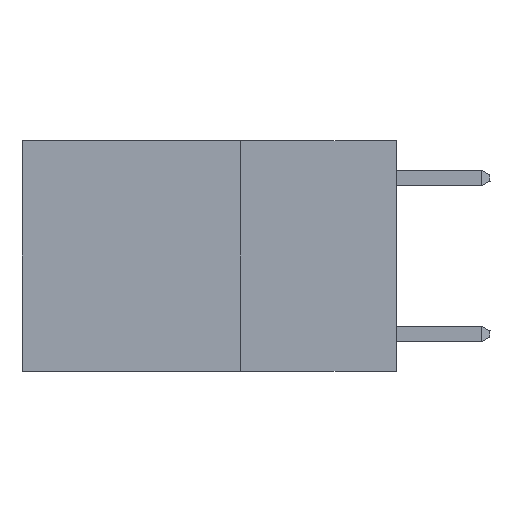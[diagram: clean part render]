
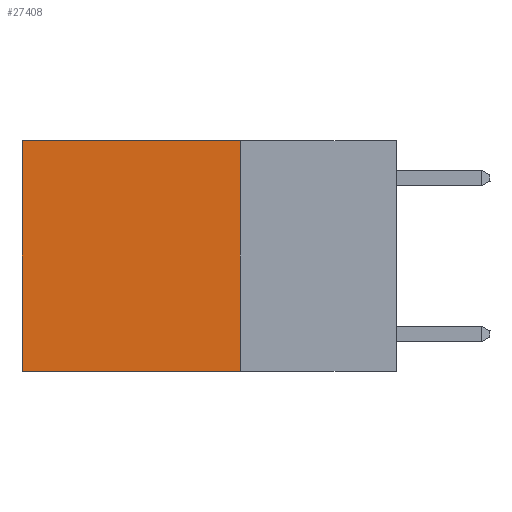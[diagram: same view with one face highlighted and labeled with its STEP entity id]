
A CAD part, left-side view. The second image highlights one B-rep face of the part: STEP entity #27408.
In plain terms, the highlighted planar face has unit normal (-1, 0, 0).
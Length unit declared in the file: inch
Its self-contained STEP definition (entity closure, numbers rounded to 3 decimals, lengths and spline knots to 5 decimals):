
#309 = VECTOR ( 'NONE', #12579, 39.37008 ) ;
#329 = DIRECTION ( 'NONE',  ( 1., 0., 0. ) ) ;
#1206 = VECTOR ( 'NONE', #25152, 39.37008 ) ;
#2781 = EDGE_CURVE ( 'NONE', #13304, #29203, #20302, .T. ) ;
#4089 = EDGE_CURVE ( 'NONE', #20739, #18573, #15946, .T. ) ;
#4998 = PLANE ( 'NONE',  #27198 ) ;
#7076 = CARTESIAN_POINT ( 'NONE',  ( 0.2625, 0.25, 0. ) ) ;
#8182 = ORIENTED_EDGE ( 'NONE', *, *, #2781, .T. ) ;
#8231 = LINE ( 'NONE', #8534, #309 ) ;
#8534 = CARTESIAN_POINT ( 'NONE',  ( 0.2625, 0.25, 0. ) ) ;
#8877 = CARTESIAN_POINT ( 'NONE',  ( 0.2625, 0.6, 0. ) ) ;
#9580 = CARTESIAN_POINT ( 'NONE',  ( 0.2625, 0.6, 0. ) ) ;
#10765 = EDGE_CURVE ( 'NONE', #18573, #29203, #24402, .T. ) ;
#11698 = CARTESIAN_POINT ( 'NONE',  ( 0.2625, 0.6, -0.37 ) ) ;
#12378 = ORIENTED_EDGE ( 'NONE', *, *, #10765, .F. ) ;
#12579 = DIRECTION ( 'NONE',  ( 0., 1., 0. ) ) ;
#13304 = VERTEX_POINT ( 'NONE', #9580 ) ;
#14966 = CARTESIAN_POINT ( 'NONE',  ( 0.2625, 0.25, 0. ) ) ;
#15522 = FACE_OUTER_BOUND ( 'NONE', #25434, .T. ) ;
#15946 = LINE ( 'NONE', #27251, #1206 ) ;
#16395 = EDGE_CURVE ( 'NONE', #20739, #13304, #8231, .T. ) ;
#17325 = DIRECTION ( 'NONE',  ( 0., 1., 0. ) ) ;
#18573 = VERTEX_POINT ( 'NONE', #19997 ) ;
#19997 = CARTESIAN_POINT ( 'NONE',  ( 0.2625, 0.25, -0.37 ) ) ;
#20302 = LINE ( 'NONE', #8877, #27061 ) ;
#20739 = VERTEX_POINT ( 'NONE', #14966 ) ;
#21335 = ORIENTED_EDGE ( 'NONE', *, *, #4089, .F. ) ;
#24011 = DIRECTION ( 'NONE',  ( 0., 0., -1. ) ) ;
#24402 = LINE ( 'NONE', #24560, #29404 ) ;
#24560 = CARTESIAN_POINT ( 'NONE',  ( 0.2625, 0.25, -0.37 ) ) ;
#25152 = DIRECTION ( 'NONE',  ( 0., 0., -1. ) ) ;
#25434 = EDGE_LOOP ( 'NONE', ( #8182, #12378, #21335, #26047 ) ) ;
#25913 = DIRECTION ( 'NONE',  ( 0., 0., -1. ) ) ;
#26047 = ORIENTED_EDGE ( 'NONE', *, *, #16395, .T. ) ;
#27061 = VECTOR ( 'NONE', #24011, 39.37008 ) ;
#27198 = AXIS2_PLACEMENT_3D ( 'NONE', #7076, #329, #25913 ) ;
#27251 = CARTESIAN_POINT ( 'NONE',  ( 0.2625, 0.25, 0. ) ) ;
#27408 = ADVANCED_FACE ( 'NONE', ( #15522 ), #4998, .F. ) ;
#29203 = VERTEX_POINT ( 'NONE', #11698 ) ;
#29404 = VECTOR ( 'NONE', #17325, 39.37008 ) ;
